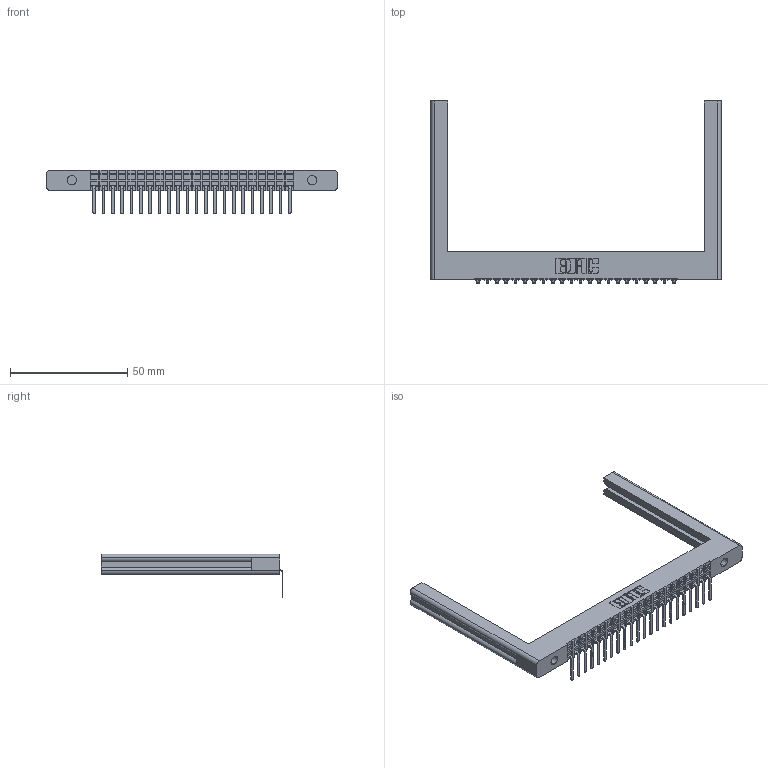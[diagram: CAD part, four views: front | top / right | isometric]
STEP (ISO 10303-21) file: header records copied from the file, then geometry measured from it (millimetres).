
FILE_DESCRIPTION (( 'STEP AP203' ), '1' );
FILE_NAME ('322-022-557-154.STEP', '2018-08-01T11:29:49', ( '' ), ( '' ), 'SwSTEP 2.0', 'SolidWorks 2016', '' );
FILE_SCHEMA (( 'CONFIG_CONTROL_DESIGN' ));
Length unit declared in the file: inch
Products named in the file (3): 322 Part; 307-290-002_557; 322-022-557-154
Assembly tree (23 placements, depth 2):
  322-022-557-154
    322 Part
    307-290-002_557  x22
Bounding box: 123.83 x 77.51 x 18.67 mm (x, y, z)
Volume: 16186.3 mm3; surface area: 19413.7 mm2
Topology: 23 solids, 23 shells, 1861 faces, 5813 edges, 3874 vertices
Faces by surface type: plane 1257, cylinder 604
Entity records: 23424 total; most frequent: ORIENTED_EDGE 4066, CARTESIAN_POINT 4056, DIRECTION 3613, EDGE_CURVE 2033, LINE 1791, VECTOR 1791, VERTEX_POINT 1354, AXIS2_PLACEMENT_3D 911
